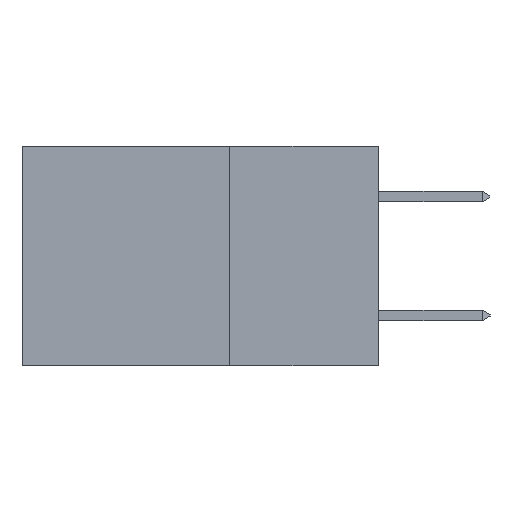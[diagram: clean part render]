
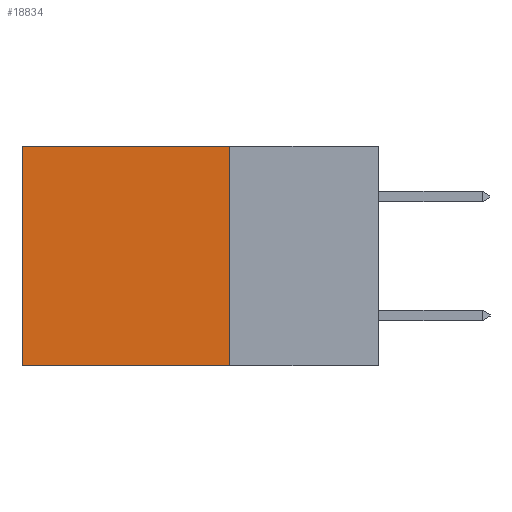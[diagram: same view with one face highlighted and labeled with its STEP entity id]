
A CAD part, left-side view. The second image highlights one B-rep face of the part: STEP entity #18834.
In plain terms, the highlighted planar face has unit normal (-1, 0, 0).
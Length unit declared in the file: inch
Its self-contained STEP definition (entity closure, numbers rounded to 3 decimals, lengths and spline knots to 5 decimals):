
#622 = PLANE ( 'NONE',  #20363 ) ;
#985 = VERTEX_POINT ( 'NONE', #17261 ) ;
#1037 = FACE_OUTER_BOUND ( 'NONE', #1520, .T. ) ;
#1520 = EDGE_LOOP ( 'NONE', ( #14600, #20644, #2546, #18579 ) ) ;
#1969 = DIRECTION ( 'NONE',  ( 0., 0., -1. ) ) ;
#2439 = CARTESIAN_POINT ( 'NONE',  ( 0.2615, 0.6, -0.37 ) ) ;
#2546 = ORIENTED_EDGE ( 'NONE', *, *, #4135, .F. ) ;
#2626 = CARTESIAN_POINT ( 'NONE',  ( 0.2615, 0.25, -0.37 ) ) ;
#2834 = CARTESIAN_POINT ( 'NONE',  ( 0.2615, 0.25, -0.37 ) ) ;
#2940 = VECTOR ( 'NONE', #6868, 39.37008 ) ;
#4017 = DIRECTION ( 'NONE',  ( 0., 0., -1. ) ) ;
#4135 = EDGE_CURVE ( 'NONE', #985, #17666, #10212, .T. ) ;
#4166 = CARTESIAN_POINT ( 'NONE',  ( 0.2615, 0.6, 0. ) ) ;
#5567 = VECTOR ( 'NONE', #5839, 39.37008 ) ;
#5796 = VECTOR ( 'NONE', #1969, 39.37008 ) ;
#5839 = DIRECTION ( 'NONE',  ( 0., 0., -1. ) ) ;
#6092 = LINE ( 'NONE', #2439, #5567 ) ;
#6868 = DIRECTION ( 'NONE',  ( 0., 1., 0. ) ) ;
#7774 = VECTOR ( 'NONE', #20486, 39.37008 ) ;
#8917 = CARTESIAN_POINT ( 'NONE',  ( 0.2615, 0.25, -0.37 ) ) ;
#9204 = VERTEX_POINT ( 'NONE', #19700 ) ;
#10204 = CARTESIAN_POINT ( 'NONE',  ( 0.2615, 0.25, 0. ) ) ;
#10212 = LINE ( 'NONE', #2626, #5796 ) ;
#11306 = LINE ( 'NONE', #10204, #2940 ) ;
#12117 = EDGE_CURVE ( 'NONE', #17666, #9204, #19424, .T. ) ;
#12364 = CARTESIAN_POINT ( 'NONE',  ( 0.2615, 0.25, -0.37 ) ) ;
#14055 = DIRECTION ( 'NONE',  ( 1., 0., 0. ) ) ;
#14600 = ORIENTED_EDGE ( 'NONE', *, *, #15312, .T. ) ;
#15023 = EDGE_CURVE ( 'NONE', #985, #19208, #11306, .T. ) ;
#15312 = EDGE_CURVE ( 'NONE', #19208, #9204, #6092, .T. ) ;
#17261 = CARTESIAN_POINT ( 'NONE',  ( 0.2615, 0.25, 0. ) ) ;
#17666 = VERTEX_POINT ( 'NONE', #2834 ) ;
#18579 = ORIENTED_EDGE ( 'NONE', *, *, #15023, .T. ) ;
#18834 = ADVANCED_FACE ( 'NONE', ( #1037 ), #622, .F. ) ;
#19208 = VERTEX_POINT ( 'NONE', #4166 ) ;
#19424 = LINE ( 'NONE', #8917, #7774 ) ;
#19700 = CARTESIAN_POINT ( 'NONE',  ( 0.2615, 0.6, -0.37 ) ) ;
#20363 = AXIS2_PLACEMENT_3D ( 'NONE', #12364, #14055, #4017 ) ;
#20486 = DIRECTION ( 'NONE',  ( 0., 1., 0. ) ) ;
#20644 = ORIENTED_EDGE ( 'NONE', *, *, #12117, .F. ) ;
